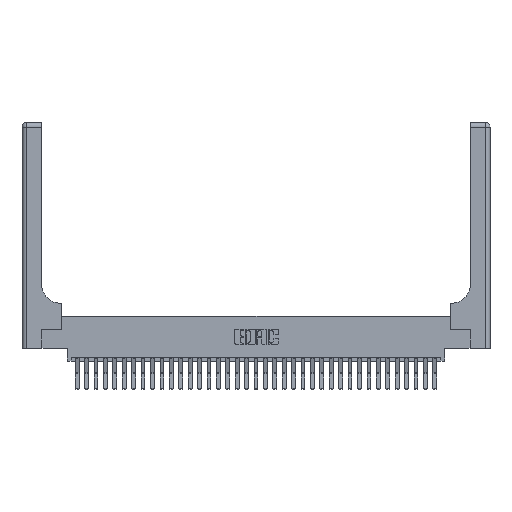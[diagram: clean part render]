
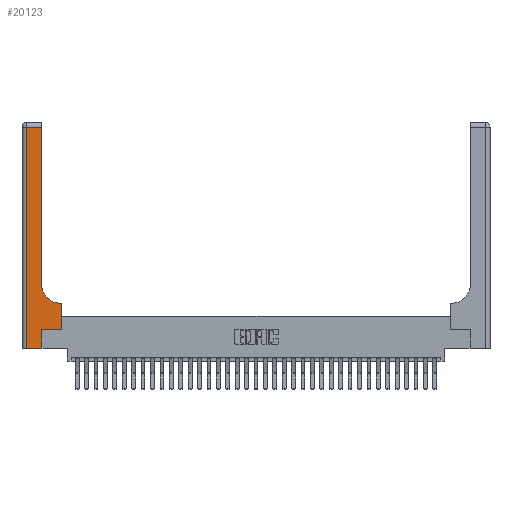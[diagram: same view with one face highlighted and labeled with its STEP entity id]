
A CAD part, top view. The second image highlights one B-rep face of the part: STEP entity #20123.
In plain terms, the highlighted planar face has unit normal (0, 0, 1).
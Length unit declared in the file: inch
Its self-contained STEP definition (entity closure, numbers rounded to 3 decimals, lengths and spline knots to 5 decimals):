
#237 = FACE_OUTER_BOUND ( 'NONE', #29172, .T. ) ;
#337 = VECTOR ( 'NONE', #5844, 39.37008 ) ;
#357 = VECTOR ( 'NONE', #370, 39.37008 ) ;
#370 = DIRECTION ( 'NONE',  ( 1., 0., 0. ) ) ;
#506 = ORIENTED_EDGE ( 'NONE', *, *, #6880, .T. ) ;
#655 = CARTESIAN_POINT ( 'NONE',  ( 0.26, 0.6, 0.37 ) ) ;
#1127 = EDGE_CURVE ( 'NONE', #12283, #12547, #6525, .T. ) ;
#1326 = DIRECTION ( 'NONE',  ( -1., 0., 0. ) ) ;
#1516 = CARTESIAN_POINT ( 'NONE',  ( 0.265, 0., 0.37 ) ) ;
#1752 = DIRECTION ( 'NONE',  ( 0., 0., -1. ) ) ;
#3067 = DIRECTION ( 'NONE',  ( -1., 0., 0. ) ) ;
#3107 = CARTESIAN_POINT ( 'NONE',  ( 0.51, 0.6, 0.37 ) ) ;
#3533 = DIRECTION ( 'NONE',  ( 0., 1., 0. ) ) ;
#3614 = VECTOR ( 'NONE', #3067, 39.37008 ) ;
#3674 = EDGE_CURVE ( 'NONE', #17416, #7513, #6774, .T. ) ;
#3974 = ORIENTED_EDGE ( 'NONE', *, *, #3674, .T. ) ;
#5404 = EDGE_CURVE ( 'NONE', #12547, #25432, #18372, .T. ) ;
#5765 = CARTESIAN_POINT ( 'NONE',  ( 0.06, 3., 0.37 ) ) ;
#5844 = DIRECTION ( 'NONE',  ( 0., 1., 0. ) ) ;
#6525 = CIRCLE ( 'NONE', #12488, 0.25 ) ;
#6774 = LINE ( 'NONE', #12984, #337 ) ;
#6880 = EDGE_CURVE ( 'NONE', #7513, #16340, #14713, .T. ) ;
#7513 = VERTEX_POINT ( 'NONE', #19343 ) ;
#8228 = DIRECTION ( 'NONE',  ( 0., -1., 0. ) ) ;
#8715 = VECTOR ( 'NONE', #3533, 39.37008 ) ;
#8745 = ORIENTED_EDGE ( 'NONE', *, *, #13767, .T. ) ;
#9341 = ORIENTED_EDGE ( 'NONE', *, *, #1127, .T. ) ;
#9621 = LINE ( 'NONE', #5765, #20954 ) ;
#10933 = CARTESIAN_POINT ( 'NONE',  ( 0.06, 0., 0.37 ) ) ;
#11310 = VERTEX_POINT ( 'NONE', #17449 ) ;
#12283 = VERTEX_POINT ( 'NONE', #3107 ) ;
#12412 = CARTESIAN_POINT ( 'NONE',  ( 0.528, 0.25, 0.37 ) ) ;
#12488 = AXIS2_PLACEMENT_3D ( 'NONE', #16202, #1752, #18636 ) ;
#12547 = VERTEX_POINT ( 'NONE', #18506 ) ;
#12984 = CARTESIAN_POINT ( 'NONE',  ( 0.265, 0., 0.37 ) ) ;
#13506 = DIRECTION ( 'NONE',  ( 1., 0., 0. ) ) ;
#13767 = EDGE_CURVE ( 'NONE', #25432, #11310, #20715, .T. ) ;
#14713 = LINE ( 'NONE', #29299, #357 ) ;
#14849 = CARTESIAN_POINT ( 'NONE',  ( 0.26, 2.94, 0.37 ) ) ;
#15121 = LINE ( 'NONE', #15570, #8715 ) ;
#15570 = CARTESIAN_POINT ( 'NONE',  ( 0.528, 0.25, 0.37 ) ) ;
#15774 = DIRECTION ( 'NONE',  ( 0., 0., -1. ) ) ;
#15802 = CARTESIAN_POINT ( 'NONE',  ( 0., 2.94, 0.37 ) ) ;
#15846 = EDGE_CURVE ( 'NONE', #16381, #12283, #16437, .T. ) ;
#15948 = CARTESIAN_POINT ( 'NONE',  ( 0., 0., 0.37 ) ) ;
#16162 = ORIENTED_EDGE ( 'NONE', *, *, #21532, .T. ) ;
#16202 = CARTESIAN_POINT ( 'NONE',  ( 0.51, 0.85, 0.37 ) ) ;
#16340 = VERTEX_POINT ( 'NONE', #12412 ) ;
#16381 = VERTEX_POINT ( 'NONE', #22258 ) ;
#16437 = LINE ( 'NONE', #655, #3614 ) ;
#16906 = CARTESIAN_POINT ( 'NONE',  ( 0.26, 3., 0.37 ) ) ;
#17416 = VERTEX_POINT ( 'NONE', #1516 ) ;
#17449 = CARTESIAN_POINT ( 'NONE',  ( 0.06, 2.94, 0.37 ) ) ;
#18112 = CARTESIAN_POINT ( 'NONE',  ( 0., 3., 0.37 ) ) ;
#18235 = DIRECTION ( 'NONE',  ( -1., 0., 0. ) ) ;
#18372 = LINE ( 'NONE', #16906, #23282 ) ;
#18506 = CARTESIAN_POINT ( 'NONE',  ( 0.26, 0.85, 0.37 ) ) ;
#18636 = DIRECTION ( 'NONE',  ( 1., 0., 0. ) ) ;
#19343 = CARTESIAN_POINT ( 'NONE',  ( 0.265, 0.25, 0.37 ) ) ;
#19954 = VECTOR ( 'NONE', #18235, 39.37008 ) ;
#20122 = VERTEX_POINT ( 'NONE', #10933 ) ;
#20123 = ADVANCED_FACE ( 'NONE', ( #237 ), #30269, .F. ) ;
#20438 = ORIENTED_EDGE ( 'NONE', *, *, #15846, .T. ) ;
#20715 = LINE ( 'NONE', #15802, #19954 ) ;
#20954 = VECTOR ( 'NONE', #8228, 39.37008 ) ;
#21532 = EDGE_CURVE ( 'NONE', #11310, #20122, #9621, .T. ) ;
#21771 = ORIENTED_EDGE ( 'NONE', *, *, #23905, .T. ) ;
#21885 = LINE ( 'NONE', #15948, #22655 ) ;
#22258 = CARTESIAN_POINT ( 'NONE',  ( 0.528, 0.6, 0.37 ) ) ;
#22633 = ORIENTED_EDGE ( 'NONE', *, *, #5404, .T. ) ;
#22655 = VECTOR ( 'NONE', #13506, 39.37008 ) ;
#23282 = VECTOR ( 'NONE', #28949, 39.37008 ) ;
#23905 = EDGE_CURVE ( 'NONE', #16340, #16381, #15121, .T. ) ;
#24593 = EDGE_CURVE ( 'NONE', #20122, #17416, #21885, .T. ) ;
#25432 = VERTEX_POINT ( 'NONE', #14849 ) ;
#28791 = ORIENTED_EDGE ( 'NONE', *, *, #24593, .T. ) ;
#28949 = DIRECTION ( 'NONE',  ( 0., 1., 0. ) ) ;
#29172 = EDGE_LOOP ( 'NONE', ( #22633, #8745, #16162, #28791, #3974, #506, #21771, #20438, #9341 ) ) ;
#29299 = CARTESIAN_POINT ( 'NONE',  ( 0.265, 0.25, 0.37 ) ) ;
#29350 = AXIS2_PLACEMENT_3D ( 'NONE', #18112, #15774, #1326 ) ;
#30269 = PLANE ( 'NONE',  #29350 ) ;
